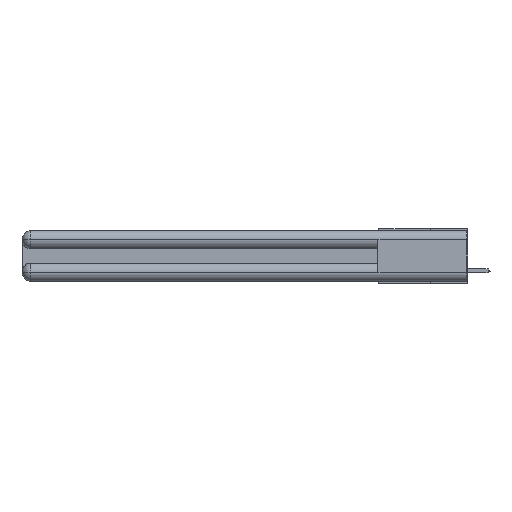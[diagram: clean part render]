
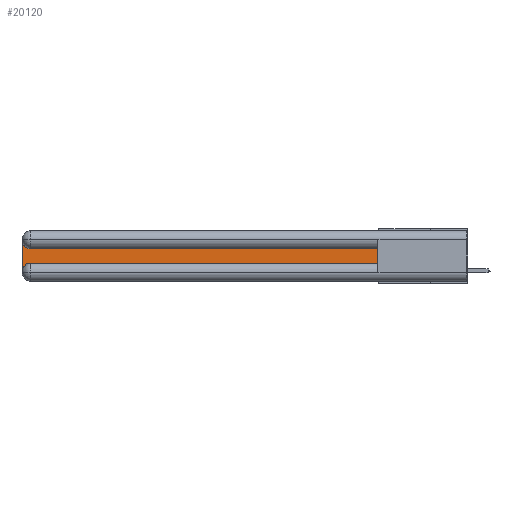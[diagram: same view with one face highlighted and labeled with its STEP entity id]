
A CAD part, left-side view. The second image highlights one B-rep face of the part: STEP entity #20120.
In plain terms, the highlighted planar face has unit normal (-1, 0, 0).
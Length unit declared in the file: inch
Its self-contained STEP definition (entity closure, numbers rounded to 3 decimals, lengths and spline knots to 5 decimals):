
#453 = VERTEX_POINT ( 'NONE', #11498 ) ;
#488 = DIRECTION ( 'NONE',  ( 0., 0., -1. ) ) ;
#1201 = EDGE_CURVE ( 'NONE', #11401, #12396, #13899, .T. ) ;
#1450 = CARTESIAN_POINT ( 'NONE',  ( 0.075, 0.6, -0.1225 ) ) ;
#2172 = VECTOR ( 'NONE', #5639, 39.37008 ) ;
#2184 = AXIS2_PLACEMENT_3D ( 'NONE', #17669, #21603, #11368 ) ;
#3063 = CARTESIAN_POINT ( 'NONE',  ( 0.075, 0.6, -0.2175 ) ) ;
#3594 = ORIENTED_EDGE ( 'NONE', *, *, #1201, .T. ) ;
#3675 = VERTEX_POINT ( 'NONE', #6369 ) ;
#4691 = DIRECTION ( 'NONE',  ( 1., 0., 0. ) ) ;
#4869 = EDGE_CURVE ( 'NONE', #19544, #18233, #11620, .T. ) ;
#5639 = DIRECTION ( 'NONE',  ( 0., -1., 0. ) ) ;
#6369 = CARTESIAN_POINT ( 'NONE',  ( 0.075, 0.6, -0.2175 ) ) ;
#7257 = PLANE ( 'NONE',  #2184 ) ;
#7356 = CARTESIAN_POINT ( 'NONE',  ( 0.075, 2.94, -0.1225 ) ) ;
#7711 = LINE ( 'NONE', #8747, #23400 ) ;
#8403 = VECTOR ( 'NONE', #22336, 39.37008 ) ;
#8747 = CARTESIAN_POINT ( 'NONE',  ( 0.075, 3., -0.2175 ) ) ;
#8840 = DIRECTION ( 'NONE',  ( 0., 0., -1. ) ) ;
#9291 = DIRECTION ( 'NONE',  ( 1., 0., 0. ) ) ;
#9995 = ORIENTED_EDGE ( 'NONE', *, *, #19896, .T. ) ;
#10448 = VECTOR ( 'NONE', #17227, 39.37008 ) ;
#10760 = FACE_OUTER_BOUND ( 'NONE', #19806, .T. ) ;
#10790 = LINE ( 'NONE', #24187, #2172 ) ;
#11170 = CARTESIAN_POINT ( 'NONE',  ( 0.075, 2.94, -0.0625 ) ) ;
#11337 = EDGE_CURVE ( 'NONE', #18233, #3675, #10790, .T. ) ;
#11368 = DIRECTION ( 'NONE',  ( 0., 0., -1. ) ) ;
#11401 = VERTEX_POINT ( 'NONE', #1450 ) ;
#11498 = CARTESIAN_POINT ( 'NONE',  ( 0.075, 3., -0.0625 ) ) ;
#11620 = CIRCLE ( 'NONE', #16373, 0.06 ) ;
#12396 = VERTEX_POINT ( 'NONE', #7356 ) ;
#13899 = LINE ( 'NONE', #24385, #8403 ) ;
#15631 = LINE ( 'NONE', #3063, #10448 ) ;
#16332 = ORIENTED_EDGE ( 'NONE', *, *, #11337, .T. ) ;
#16373 = AXIS2_PLACEMENT_3D ( 'NONE', #25290, #4691, #488 ) ;
#17227 = DIRECTION ( 'NONE',  ( 0., 0., 1. ) ) ;
#17669 = CARTESIAN_POINT ( 'NONE',  ( 0.075, 3., -0.1225 ) ) ;
#17805 = CARTESIAN_POINT ( 'NONE',  ( 0.075, 2.94, -0.2175 ) ) ;
#18233 = VERTEX_POINT ( 'NONE', #17805 ) ;
#18549 = AXIS2_PLACEMENT_3D ( 'NONE', #11170, #9291, #19347 ) ;
#18995 = ORIENTED_EDGE ( 'NONE', *, *, #24884, .T. ) ;
#19347 = DIRECTION ( 'NONE',  ( 0., 0., -1. ) ) ;
#19544 = VERTEX_POINT ( 'NONE', #21568 ) ;
#19806 = EDGE_LOOP ( 'NONE', ( #3594, #18995, #26260, #25786, #16332, #9995 ) ) ;
#19896 = EDGE_CURVE ( 'NONE', #3675, #11401, #15631, .T. ) ;
#20120 = ADVANCED_FACE ( 'NONE', ( #10760 ), #7257, .F. ) ;
#21096 = CIRCLE ( 'NONE', #18549, 0.06 ) ;
#21568 = CARTESIAN_POINT ( 'NONE',  ( 0.075, 3., -0.2775 ) ) ;
#21603 = DIRECTION ( 'NONE',  ( 1., 0., 0. ) ) ;
#22336 = DIRECTION ( 'NONE',  ( 0., 1., 0. ) ) ;
#23400 = VECTOR ( 'NONE', #8840, 39.37008 ) ;
#23763 = EDGE_CURVE ( 'NONE', #453, #19544, #7711, .T. ) ;
#24187 = CARTESIAN_POINT ( 'NONE',  ( 0.075, 0.6, -0.2175 ) ) ;
#24385 = CARTESIAN_POINT ( 'NONE',  ( 0.075, 0.6, -0.1225 ) ) ;
#24884 = EDGE_CURVE ( 'NONE', #12396, #453, #21096, .T. ) ;
#25290 = CARTESIAN_POINT ( 'NONE',  ( 0.075, 2.94, -0.2775 ) ) ;
#25786 = ORIENTED_EDGE ( 'NONE', *, *, #4869, .T. ) ;
#26260 = ORIENTED_EDGE ( 'NONE', *, *, #23763, .T. ) ;
